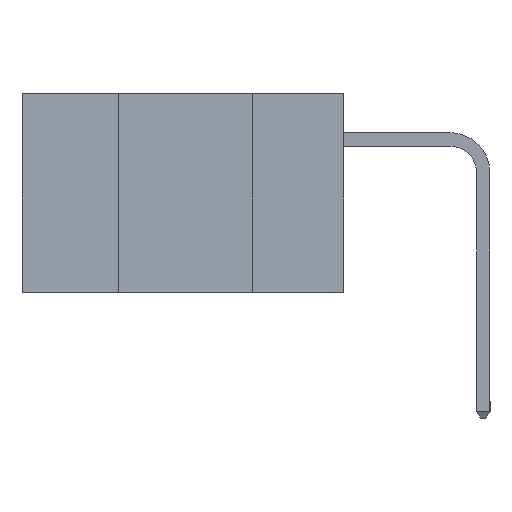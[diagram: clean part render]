
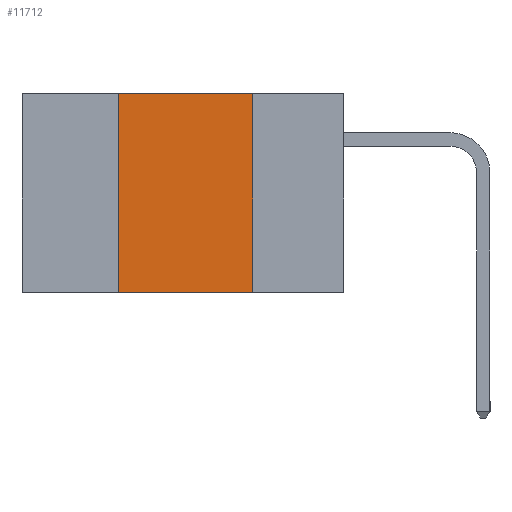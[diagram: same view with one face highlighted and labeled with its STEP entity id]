
A CAD part, left-side view. The second image highlights one B-rep face of the part: STEP entity #11712.
In plain terms, the highlighted planar face has unit normal (-1, 0, 0).
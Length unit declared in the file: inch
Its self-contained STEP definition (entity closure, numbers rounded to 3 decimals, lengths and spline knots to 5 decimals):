
#623 = CARTESIAN_POINT ( 'NONE',  ( 0., 0.6, 0. ) ) ;
#900 = LINE ( 'NONE', #623, #12408 ) ;
#1371 = EDGE_CURVE ( 'NONE', #11626, #1696, #14583, .T. ) ;
#1696 = VERTEX_POINT ( 'NONE', #3102 ) ;
#2124 = DIRECTION ( 'NONE',  ( 0., -1., 0. ) ) ;
#2545 = VECTOR ( 'NONE', #14469, 39.37008 ) ;
#3102 = CARTESIAN_POINT ( 'NONE',  ( 0., 0.17, -0.37 ) ) ;
#4397 = EDGE_CURVE ( 'NONE', #11626, #7781, #14711, .T. ) ;
#4995 = CARTESIAN_POINT ( 'NONE',  ( 0., 0.42, 0. ) ) ;
#5185 = ORIENTED_EDGE ( 'NONE', *, *, #12589, .F. ) ;
#5258 = EDGE_LOOP ( 'NONE', ( #5185, #17636, #6126, #18538 ) ) ;
#6031 = VERTEX_POINT ( 'NONE', #6324 ) ;
#6126 = ORIENTED_EDGE ( 'NONE', *, *, #4397, .F. ) ;
#6324 = CARTESIAN_POINT ( 'NONE',  ( 0., 0.17, 0. ) ) ;
#7781 = VERTEX_POINT ( 'NONE', #4995 ) ;
#9445 = DIRECTION ( 'NONE',  ( 0., 0., -1. ) ) ;
#9590 = LINE ( 'NONE', #9628, #13597 ) ;
#9628 = CARTESIAN_POINT ( 'NONE',  ( 0., 0.17, -0.37 ) ) ;
#10004 = DIRECTION ( 'NONE',  ( 0., 0., -1. ) ) ;
#10047 = DIRECTION ( 'NONE',  ( 1., 0., 0. ) ) ;
#10065 = CARTESIAN_POINT ( 'NONE',  ( 0., 0.6, 0. ) ) ;
#10230 = VECTOR ( 'NONE', #11081, 39.37008 ) ;
#10766 = PLANE ( 'NONE',  #15337 ) ;
#11017 = CARTESIAN_POINT ( 'NONE',  ( 0., 0.42, -0.37 ) ) ;
#11081 = DIRECTION ( 'NONE',  ( 0., 0., 1. ) ) ;
#11626 = VERTEX_POINT ( 'NONE', #11671 ) ;
#11671 = CARTESIAN_POINT ( 'NONE',  ( 0., 0.42, -0.37 ) ) ;
#11712 = ADVANCED_FACE ( 'NONE', ( #16688 ), #10766, .F. ) ;
#12408 = VECTOR ( 'NONE', #2124, 39.37008 ) ;
#12589 = EDGE_CURVE ( 'NONE', #6031, #1696, #9590, .T. ) ;
#13597 = VECTOR ( 'NONE', #9445, 39.37008 ) ;
#14469 = DIRECTION ( 'NONE',  ( 0., -1., 0. ) ) ;
#14511 = CARTESIAN_POINT ( 'NONE',  ( 0., 0.6, -0.37 ) ) ;
#14583 = LINE ( 'NONE', #14511, #2545 ) ;
#14711 = LINE ( 'NONE', #11017, #10230 ) ;
#15337 = AXIS2_PLACEMENT_3D ( 'NONE', #10065, #10047, #10004 ) ;
#16133 = EDGE_CURVE ( 'NONE', #7781, #6031, #900, .T. ) ;
#16688 = FACE_OUTER_BOUND ( 'NONE', #5258, .T. ) ;
#17636 = ORIENTED_EDGE ( 'NONE', *, *, #16133, .F. ) ;
#18538 = ORIENTED_EDGE ( 'NONE', *, *, #1371, .T. ) ;
